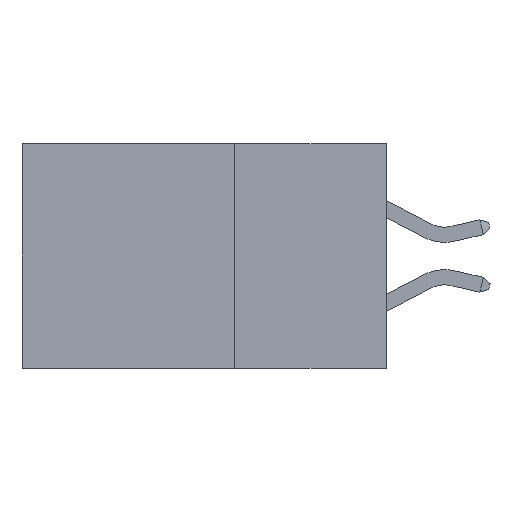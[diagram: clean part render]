
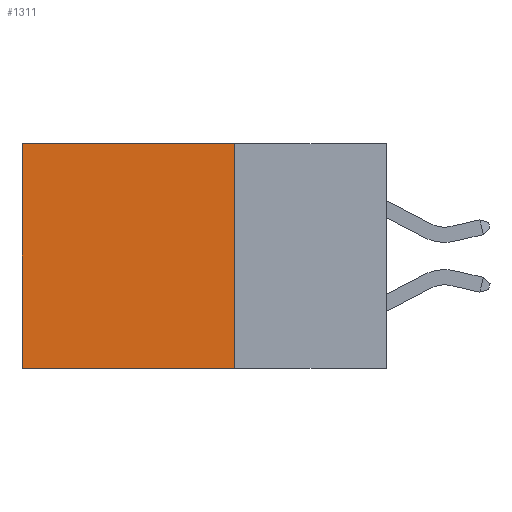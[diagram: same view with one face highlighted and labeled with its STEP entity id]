
A CAD part, left-side view. The second image highlights one B-rep face of the part: STEP entity #1311.
In plain terms, the highlighted planar face has unit normal (-1, 0, 0).
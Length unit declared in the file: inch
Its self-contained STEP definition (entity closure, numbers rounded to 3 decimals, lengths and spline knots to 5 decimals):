
#9 = CARTESIAN_POINT ( 'NONE',  ( 0.298, 0.25, 0. ) ) ;
#980 = ORIENTED_EDGE ( 'NONE', *, *, #2496, .T. ) ;
#1311 = ADVANCED_FACE ( 'NONE', ( #22710 ), #21246, .F. ) ;
#1723 = VECTOR ( 'NONE', #28995, 39.37008 ) ;
#2496 = EDGE_CURVE ( 'NONE', #5814, #10965, #10610, .T. ) ;
#3280 = EDGE_CURVE ( 'NONE', #3994, #18202, #23488, .T. ) ;
#3730 = DIRECTION ( 'NONE',  ( 0., 1., 0. ) ) ;
#3994 = VERTEX_POINT ( 'NONE', #4819 ) ;
#4080 = AXIS2_PLACEMENT_3D ( 'NONE', #23521, #9824, #25827 ) ;
#4466 = DIRECTION ( 'NONE',  ( 0., 1., 0. ) ) ;
#4819 = CARTESIAN_POINT ( 'NONE',  ( 0.298, 0.25, -0.37 ) ) ;
#5814 = VERTEX_POINT ( 'NONE', #9 ) ;
#8231 = EDGE_LOOP ( 'NONE', ( #23708, #14428, #12492, #980 ) ) ;
#9824 = DIRECTION ( 'NONE',  ( 1., 0., 0. ) ) ;
#9959 = CARTESIAN_POINT ( 'NONE',  ( 0.298, 0.6, 0. ) ) ;
#10610 = LINE ( 'NONE', #24264, #26350 ) ;
#10644 = CARTESIAN_POINT ( 'NONE',  ( 0.298, 0.6, 0. ) ) ;
#10965 = VERTEX_POINT ( 'NONE', #9959 ) ;
#11041 = EDGE_CURVE ( 'NONE', #10965, #18202, #20721, .T. ) ;
#12492 = ORIENTED_EDGE ( 'NONE', *, *, #18876, .F. ) ;
#13548 = DIRECTION ( 'NONE',  ( 0., 0., -1. ) ) ;
#14428 = ORIENTED_EDGE ( 'NONE', *, *, #3280, .F. ) ;
#15988 = CARTESIAN_POINT ( 'NONE',  ( 0.298, 0.6, -0.37 ) ) ;
#18202 = VERTEX_POINT ( 'NONE', #15988 ) ;
#18836 = VECTOR ( 'NONE', #4466, 39.37008 ) ;
#18876 = EDGE_CURVE ( 'NONE', #5814, #3994, #25553, .T. ) ;
#19457 = VECTOR ( 'NONE', #13548, 39.37008 ) ;
#20721 = LINE ( 'NONE', #10644, #1723 ) ;
#21246 = PLANE ( 'NONE',  #4080 ) ;
#22710 = FACE_OUTER_BOUND ( 'NONE', #8231, .T. ) ;
#22981 = CARTESIAN_POINT ( 'NONE',  ( 0.298, 0.25, -0.37 ) ) ;
#23488 = LINE ( 'NONE', #22981, #18836 ) ;
#23521 = CARTESIAN_POINT ( 'NONE',  ( 0.298, 0.25, 0. ) ) ;
#23708 = ORIENTED_EDGE ( 'NONE', *, *, #11041, .T. ) ;
#24264 = CARTESIAN_POINT ( 'NONE',  ( 0.298, 0.25, 0. ) ) ;
#24765 = CARTESIAN_POINT ( 'NONE',  ( 0.298, 0.25, 0. ) ) ;
#25553 = LINE ( 'NONE', #24765, #19457 ) ;
#25827 = DIRECTION ( 'NONE',  ( 0., 0., -1. ) ) ;
#26350 = VECTOR ( 'NONE', #3730, 39.37008 ) ;
#28995 = DIRECTION ( 'NONE',  ( 0., 0., -1. ) ) ;
